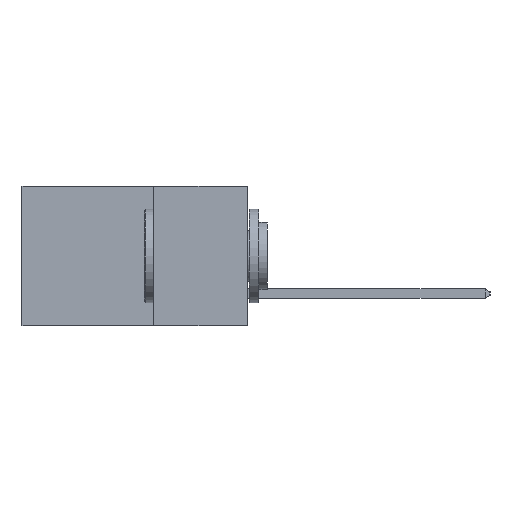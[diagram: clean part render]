
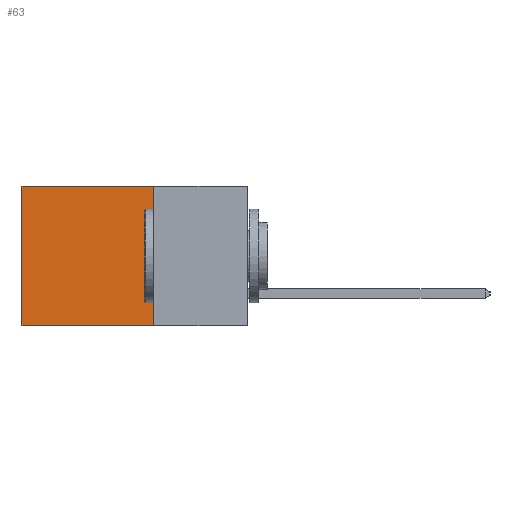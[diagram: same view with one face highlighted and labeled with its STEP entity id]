
A CAD part, left-side view. The second image highlights one B-rep face of the part: STEP entity #63.
In plain terms, the highlighted planar face has unit normal (-1, 0, 0).
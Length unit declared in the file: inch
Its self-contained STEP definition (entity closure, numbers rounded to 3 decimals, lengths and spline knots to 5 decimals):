
#63 = ADVANCED_FACE ( 'NONE', ( #13241 ), #5991, .F. ) ;
#436 = DIRECTION ( 'NONE',  ( 1., 0., 0. ) ) ;
#447 = LINE ( 'NONE', #6448, #4066 ) ;
#1281 = LINE ( 'NONE', #4084, #2127 ) ;
#1307 = VECTOR ( 'NONE', #3857, 39.37008 ) ;
#1897 = VERTEX_POINT ( 'NONE', #5292 ) ;
#2127 = VECTOR ( 'NONE', #13993, 39.37008 ) ;
#2350 = ORIENTED_EDGE ( 'NONE', *, *, #9967, .T. ) ;
#2582 = VECTOR ( 'NONE', #4681, 39.37008 ) ;
#2622 = CARTESIAN_POINT ( 'NONE',  ( 0.2615, 0.25, -0.37 ) ) ;
#2626 = CARTESIAN_POINT ( 'NONE',  ( 0.2615, 0.6, 0. ) ) ;
#3365 = CARTESIAN_POINT ( 'NONE',  ( 0.2615, 0.25, -0.37 ) ) ;
#3638 = ORIENTED_EDGE ( 'NONE', *, *, #6086, .F. ) ;
#3750 = EDGE_CURVE ( 'NONE', #4741, #10239, #1281, .T. ) ;
#3857 = DIRECTION ( 'NONE',  ( 0., 0., -1. ) ) ;
#4066 = VECTOR ( 'NONE', #5207, 39.37008 ) ;
#4084 = CARTESIAN_POINT ( 'NONE',  ( 0.2615, 0.25, 0. ) ) ;
#4681 = DIRECTION ( 'NONE',  ( 0., 1., 0. ) ) ;
#4741 = VERTEX_POINT ( 'NONE', #8493 ) ;
#4912 = LINE ( 'NONE', #10451, #1307 ) ;
#5207 = DIRECTION ( 'NONE',  ( 0., 0., -1. ) ) ;
#5292 = CARTESIAN_POINT ( 'NONE',  ( 0.2615, 0.6, -0.37 ) ) ;
#5304 = LINE ( 'NONE', #2622, #2582 ) ;
#5991 = PLANE ( 'NONE',  #7659 ) ;
#6086 = EDGE_CURVE ( 'NONE', #12208, #1897, #5304, .T. ) ;
#6448 = CARTESIAN_POINT ( 'NONE',  ( 0.2615, 0.25, -0.37 ) ) ;
#7659 = AXIS2_PLACEMENT_3D ( 'NONE', #13756, #436, #11476 ) ;
#8355 = ORIENTED_EDGE ( 'NONE', *, *, #9034, .F. ) ;
#8493 = CARTESIAN_POINT ( 'NONE',  ( 0.2615, 0.25, 0. ) ) ;
#9034 = EDGE_CURVE ( 'NONE', #4741, #12208, #447, .T. ) ;
#9967 = EDGE_CURVE ( 'NONE', #10239, #1897, #4912, .T. ) ;
#10239 = VERTEX_POINT ( 'NONE', #2626 ) ;
#10451 = CARTESIAN_POINT ( 'NONE',  ( 0.2615, 0.6, -0.37 ) ) ;
#11476 = DIRECTION ( 'NONE',  ( 0., 0., -1. ) ) ;
#11620 = ORIENTED_EDGE ( 'NONE', *, *, #3750, .T. ) ;
#12208 = VERTEX_POINT ( 'NONE', #3365 ) ;
#13156 = EDGE_LOOP ( 'NONE', ( #2350, #3638, #8355, #11620 ) ) ;
#13241 = FACE_OUTER_BOUND ( 'NONE', #13156, .T. ) ;
#13756 = CARTESIAN_POINT ( 'NONE',  ( 0.2615, 0.25, -0.37 ) ) ;
#13993 = DIRECTION ( 'NONE',  ( 0., 1., 0. ) ) ;
